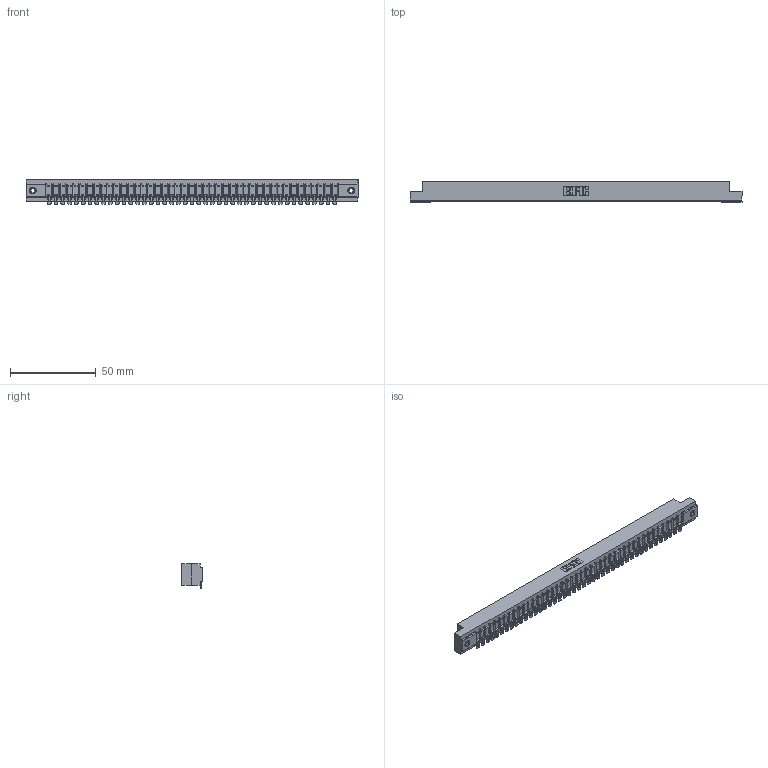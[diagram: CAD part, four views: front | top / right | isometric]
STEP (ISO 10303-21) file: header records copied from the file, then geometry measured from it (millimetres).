
FILE_DESCRIPTION (( 'STEP AP203' ), '1' );
FILE_NAME ('307-043-554-108.STEP', '2018-08-06T00:59:52', ( '' ), ( '' ), 'SwSTEP 2.0', 'SolidWorks 2016', '' );
FILE_SCHEMA (( 'CONFIG_CONTROL_DESIGN' ));
Length unit declared in the file: inch
Products named in the file (4): 307 Part_.156 Dia Mounting Holes; 307-290-002_554; 345-250-001_345-250-003-102; 307-043-554-108
Assembly tree (46 placements, depth 2):
  307-043-554-108
    307 Part_.156 Dia Mounting Holes
    307-290-002_554  x43
    345-250-001_345-250-003-102  x2
Bounding box: 193.4 x 12.01 x 14.52 mm (x, y, z)
Volume: 20712.2 mm3; surface area: 26249.7 mm2
Topology: 46 solids, 46 shells, 3705 faces, 11338 edges, 7432 vertices
Faces by surface type: plane 2080, cylinder 1521, sphere 88, cone 12, torus 4
Entity records: 38890 total; most frequent: CARTESIAN_POINT 6541, ORIENTED_EDGE 6524, DIRECTION 6370, EDGE_CURVE 3262, LINE 2492, VECTOR 2492, VERTEX_POINT 2110, AXIS2_PLACEMENT_3D 1939
